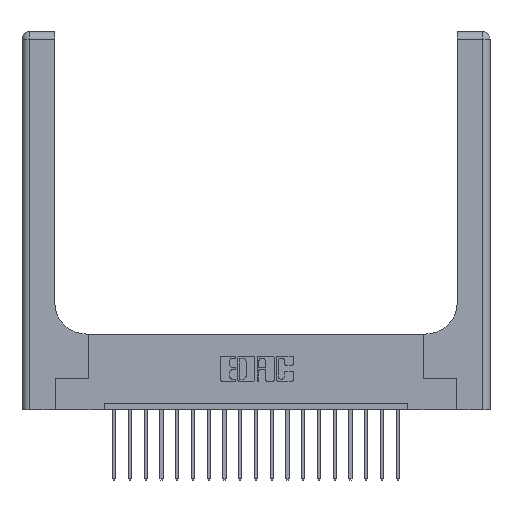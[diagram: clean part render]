
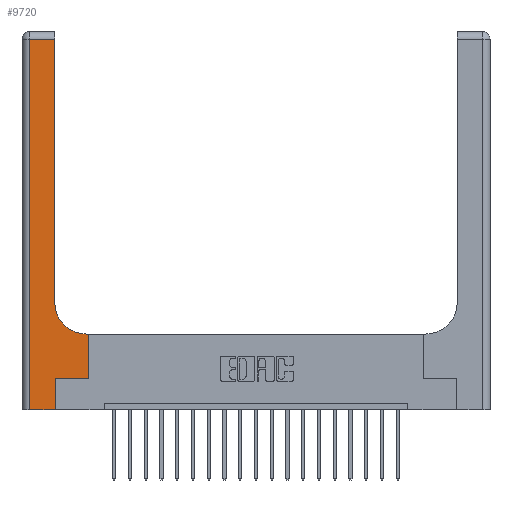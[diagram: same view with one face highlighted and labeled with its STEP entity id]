
A CAD part, top view. The second image highlights one B-rep face of the part: STEP entity #9720.
In plain terms, the highlighted planar face has unit normal (0, 0, 1).
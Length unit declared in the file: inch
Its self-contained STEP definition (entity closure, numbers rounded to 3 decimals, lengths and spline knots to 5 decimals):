
#133 = CARTESIAN_POINT ( 'NONE',  ( 0.26, 0.85, 0.37 ) ) ;
#411 = CARTESIAN_POINT ( 'NONE',  ( 0.265, 0.25, 0.37 ) ) ;
#734 = VERTEX_POINT ( 'NONE', #10777 ) ;
#1258 = CARTESIAN_POINT ( 'NONE',  ( 0.51, 0.85, 0.37 ) ) ;
#1398 = ORIENTED_EDGE ( 'NONE', *, *, #16674, .T. ) ;
#1698 = DIRECTION ( 'NONE',  ( -1., 0., 0. ) ) ;
#1833 = DIRECTION ( 'NONE',  ( 1., 0., 0. ) ) ;
#1865 = VECTOR ( 'NONE', #15580, 39.37008 ) ;
#1882 = ORIENTED_EDGE ( 'NONE', *, *, #16561, .T. ) ;
#1920 = VECTOR ( 'NONE', #4079, 39.37008 ) ;
#2441 = LINE ( 'NONE', #20121, #15200 ) ;
#2778 = VERTEX_POINT ( 'NONE', #18567 ) ;
#2916 = LINE ( 'NONE', #7911, #1865 ) ;
#2962 = EDGE_CURVE ( 'NONE', #15752, #13076, #6855, .T. ) ;
#2987 = VERTEX_POINT ( 'NONE', #10334 ) ;
#2993 = ORIENTED_EDGE ( 'NONE', *, *, #20016, .T. ) ;
#3206 = VERTEX_POINT ( 'NONE', #7968 ) ;
#3375 = FACE_OUTER_BOUND ( 'NONE', #14302, .T. ) ;
#3610 = CIRCLE ( 'NONE', #5285, 0.25 ) ;
#4079 = DIRECTION ( 'NONE',  ( 1., 0., 0. ) ) ;
#4487 = LINE ( 'NONE', #7310, #1920 ) ;
#5285 = AXIS2_PLACEMENT_3D ( 'NONE', #1258, #12965, #1833 ) ;
#6234 = DIRECTION ( 'NONE',  ( -1., 0., 0. ) ) ;
#6446 = DIRECTION ( 'NONE',  ( 0., 1., 0. ) ) ;
#6487 = EDGE_CURVE ( 'NONE', #12664, #2987, #7776, .T. ) ;
#6855 = LINE ( 'NONE', #16479, #16754 ) ;
#7310 = CARTESIAN_POINT ( 'NONE',  ( 0., 0., 0.37 ) ) ;
#7539 = CARTESIAN_POINT ( 'NONE',  ( 0.528, 0.25, 0.37 ) ) ;
#7695 = LINE ( 'NONE', #7894, #17392 ) ;
#7776 = LINE ( 'NONE', #20433, #16391 ) ;
#7785 = ORIENTED_EDGE ( 'NONE', *, *, #6487, .T. ) ;
#7833 = ORIENTED_EDGE ( 'NONE', *, *, #2962, .T. ) ;
#7894 = CARTESIAN_POINT ( 'NONE',  ( 0.265, 0., 0.37 ) ) ;
#7911 = CARTESIAN_POINT ( 'NONE',  ( 0.26, 0.6, 0.37 ) ) ;
#7968 = CARTESIAN_POINT ( 'NONE',  ( 0.51, 0.6, 0.37 ) ) ;
#8481 = VECTOR ( 'NONE', #18611, 39.37008 ) ;
#9125 = CARTESIAN_POINT ( 'NONE',  ( 0.26, 2.94, 0.37 ) ) ;
#9177 = LINE ( 'NONE', #16863, #12257 ) ;
#9373 = ORIENTED_EDGE ( 'NONE', *, *, #14304, .T. ) ;
#9720 = ADVANCED_FACE ( 'NONE', ( #3375 ), #16347, .F. ) ;
#10023 = DIRECTION ( 'NONE',  ( 1., 0., 0. ) ) ;
#10332 = EDGE_CURVE ( 'NONE', #2778, #15752, #7695, .T. ) ;
#10334 = CARTESIAN_POINT ( 'NONE',  ( 0.06, 2.94, 0.37 ) ) ;
#10777 = CARTESIAN_POINT ( 'NONE',  ( 0.06, 0., 0.37 ) ) ;
#11860 = CARTESIAN_POINT ( 'NONE',  ( 0.528, 0.6, 0.37 ) ) ;
#12257 = VECTOR ( 'NONE', #15602, 39.37008 ) ;
#12664 = VERTEX_POINT ( 'NONE', #9125 ) ;
#12965 = DIRECTION ( 'NONE',  ( 0., 0., -1. ) ) ;
#13076 = VERTEX_POINT ( 'NONE', #19689 ) ;
#13596 = EDGE_CURVE ( 'NONE', #13076, #19855, #15093, .T. ) ;
#13868 = VERTEX_POINT ( 'NONE', #133 ) ;
#14302 = EDGE_LOOP ( 'NONE', ( #2993, #7785, #16764, #1882, #19177, #7833, #19900, #9373, #1398 ) ) ;
#14304 = EDGE_CURVE ( 'NONE', #19855, #3206, #2916, .T. ) ;
#14725 = AXIS2_PLACEMENT_3D ( 'NONE', #16154, #17595, #1698 ) ;
#15093 = LINE ( 'NONE', #7539, #8481 ) ;
#15200 = VECTOR ( 'NONE', #15339, 39.37008 ) ;
#15339 = DIRECTION ( 'NONE',  ( 0., -1., 0. ) ) ;
#15580 = DIRECTION ( 'NONE',  ( -1., 0., 0. ) ) ;
#15602 = DIRECTION ( 'NONE',  ( 0., 1., 0. ) ) ;
#15752 = VERTEX_POINT ( 'NONE', #411 ) ;
#16114 = EDGE_CURVE ( 'NONE', #2987, #734, #2441, .T. ) ;
#16154 = CARTESIAN_POINT ( 'NONE',  ( 0., 3., 0.37 ) ) ;
#16347 = PLANE ( 'NONE',  #14725 ) ;
#16391 = VECTOR ( 'NONE', #6234, 39.37008 ) ;
#16479 = CARTESIAN_POINT ( 'NONE',  ( 0.265, 0.25, 0.37 ) ) ;
#16561 = EDGE_CURVE ( 'NONE', #734, #2778, #4487, .T. ) ;
#16674 = EDGE_CURVE ( 'NONE', #3206, #13868, #3610, .T. ) ;
#16754 = VECTOR ( 'NONE', #10023, 39.37008 ) ;
#16764 = ORIENTED_EDGE ( 'NONE', *, *, #16114, .T. ) ;
#16863 = CARTESIAN_POINT ( 'NONE',  ( 0.26, 3., 0.37 ) ) ;
#17392 = VECTOR ( 'NONE', #6446, 39.37008 ) ;
#17595 = DIRECTION ( 'NONE',  ( 0., 0., -1. ) ) ;
#18567 = CARTESIAN_POINT ( 'NONE',  ( 0.265, 0., 0.37 ) ) ;
#18611 = DIRECTION ( 'NONE',  ( 0., 1., 0. ) ) ;
#19177 = ORIENTED_EDGE ( 'NONE', *, *, #10332, .T. ) ;
#19689 = CARTESIAN_POINT ( 'NONE',  ( 0.528, 0.25, 0.37 ) ) ;
#19855 = VERTEX_POINT ( 'NONE', #11860 ) ;
#19900 = ORIENTED_EDGE ( 'NONE', *, *, #13596, .T. ) ;
#20016 = EDGE_CURVE ( 'NONE', #13868, #12664, #9177, .T. ) ;
#20121 = CARTESIAN_POINT ( 'NONE',  ( 0.06, 3., 0.37 ) ) ;
#20433 = CARTESIAN_POINT ( 'NONE',  ( 0., 2.94, 0.37 ) ) ;
